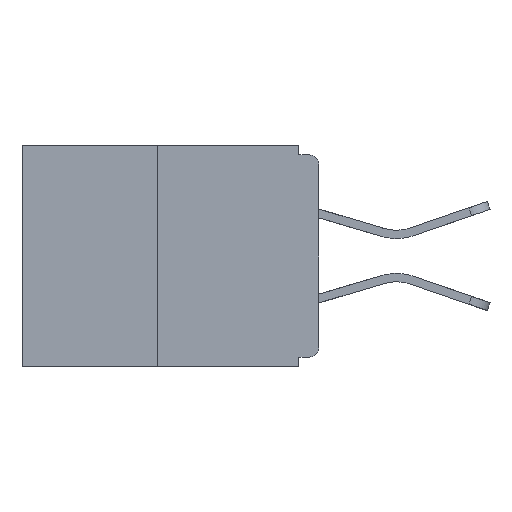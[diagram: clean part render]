
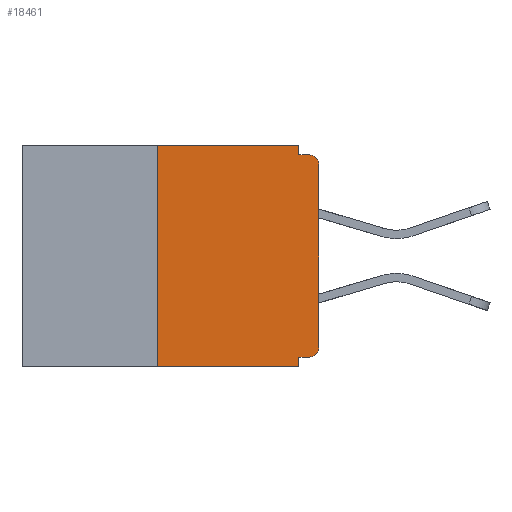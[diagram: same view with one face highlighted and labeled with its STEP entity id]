
A CAD part, left-side view. The second image highlights one B-rep face of the part: STEP entity #18461.
In plain terms, the highlighted planar face has unit normal (-1, 0, 0).
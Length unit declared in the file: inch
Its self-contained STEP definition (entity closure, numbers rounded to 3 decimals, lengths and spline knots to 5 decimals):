
#294 = VECTOR ( 'NONE', #12184, 39.37008 ) ;
#397 = VERTEX_POINT ( 'NONE', #10981 ) ;
#531 = CARTESIAN_POINT ( 'NONE',  ( 0., 0.46, -0.343 ) ) ;
#727 = LINE ( 'NONE', #11934, #294 ) ;
#805 = ORIENTED_EDGE ( 'NONE', *, *, #8348, .F. ) ;
#1010 = LINE ( 'NONE', #9107, #17300 ) ;
#1105 = DIRECTION ( 'NONE',  ( 0., 1., 0. ) ) ;
#1230 = DIRECTION ( 'NONE',  ( 0., 0., -1. ) ) ;
#1686 = DIRECTION ( 'NONE',  ( 0., 0., -1. ) ) ;
#1847 = ORIENTED_EDGE ( 'NONE', *, *, #14572, .F. ) ;
#2131 = ORIENTED_EDGE ( 'NONE', *, *, #13245, .F. ) ;
#2386 = VECTOR ( 'NONE', #1230, 39.37008 ) ;
#3093 = DIRECTION ( 'NONE',  ( 0., 0., -1. ) ) ;
#3113 = CARTESIAN_POINT ( 'NONE',  ( 0., 0.46, 0. ) ) ;
#3115 = VERTEX_POINT ( 'NONE', #5912 ) ;
#3250 = CARTESIAN_POINT ( 'NONE',  ( 0., 0.031, -0.015 ) ) ;
#3335 = VERTEX_POINT ( 'NONE', #14692 ) ;
#3386 = VERTEX_POINT ( 'NONE', #14561 ) ;
#3626 = VECTOR ( 'NONE', #14901, 39.37008 ) ;
#3733 = CARTESIAN_POINT ( 'NONE',  ( 0., 0.25, 0. ) ) ;
#4207 = LINE ( 'NONE', #9848, #2386 ) ;
#4228 = CIRCLE ( 'NONE', #4556, 0.015 ) ;
#4556 = AXIS2_PLACEMENT_3D ( 'NONE', #13564, #6342, #10470 ) ;
#4960 = DIRECTION ( 'NONE',  ( 0., -1., 0. ) ) ;
#5439 = VERTEX_POINT ( 'NONE', #5561 ) ;
#5561 = CARTESIAN_POINT ( 'NONE',  ( 0., 0.25, 0. ) ) ;
#5897 = EDGE_CURVE ( 'NONE', #17363, #3386, #16317, .T. ) ;
#5912 = CARTESIAN_POINT ( 'NONE',  ( 0., 0.015, -0.015 ) ) ;
#6247 = EDGE_CURVE ( 'NONE', #5439, #13983, #18509, .T. ) ;
#6342 = DIRECTION ( 'NONE',  ( -1., 0., 0. ) ) ;
#6622 = DIRECTION ( 'NONE',  ( 0., 0., 1. ) ) ;
#6623 = ORIENTED_EDGE ( 'NONE', *, *, #11339, .T. ) ;
#6711 = CARTESIAN_POINT ( 'NONE',  ( 0., 0.031, -0.328 ) ) ;
#6913 = VECTOR ( 'NONE', #1105, 39.37008 ) ;
#7054 = ORIENTED_EDGE ( 'NONE', *, *, #7511, .T. ) ;
#7511 = EDGE_CURVE ( 'NONE', #11652, #397, #8540, .T. ) ;
#8054 = CIRCLE ( 'NONE', #11321, 0.015 ) ;
#8132 = FACE_OUTER_BOUND ( 'NONE', #16042, .T. ) ;
#8278 = DIRECTION ( 'NONE',  ( 0., 0., 1. ) ) ;
#8348 = EDGE_CURVE ( 'NONE', #16678, #3115, #727, .T. ) ;
#8540 = LINE ( 'NONE', #531, #3626 ) ;
#8627 = CARTESIAN_POINT ( 'NONE',  ( 0., 0.015, -0.313 ) ) ;
#8867 = DIRECTION ( 'NONE',  ( -1., 0., 0. ) ) ;
#9107 = CARTESIAN_POINT ( 'NONE',  ( 0., 0.031, -0.343 ) ) ;
#9405 = EDGE_CURVE ( 'NONE', #11652, #5439, #13997, .T. ) ;
#9811 = CARTESIAN_POINT ( 'NONE',  ( 0., 0.25, -0.343 ) ) ;
#9848 = CARTESIAN_POINT ( 'NONE',  ( 0., 0.031, 0. ) ) ;
#10288 = PLANE ( 'NONE',  #15900 ) ;
#10373 = VECTOR ( 'NONE', #6622, 39.37008 ) ;
#10470 = DIRECTION ( 'NONE',  ( 0., 0., -1. ) ) ;
#10788 = ORIENTED_EDGE ( 'NONE', *, *, #14985, .F. ) ;
#10981 = CARTESIAN_POINT ( 'NONE',  ( 0., 0.031, -0.343 ) ) ;
#11066 = VECTOR ( 'NONE', #4960, 39.37008 ) ;
#11321 = AXIS2_PLACEMENT_3D ( 'NONE', #8627, #8867, #3093 ) ;
#11339 = EDGE_CURVE ( 'NONE', #3386, #3115, #4228, .T. ) ;
#11652 = VERTEX_POINT ( 'NONE', #9811 ) ;
#11829 = CARTESIAN_POINT ( 'NONE',  ( 0., 0., -0.313 ) ) ;
#11934 = CARTESIAN_POINT ( 'NONE',  ( 0., 0., -0.015 ) ) ;
#12066 = DIRECTION ( 'NONE',  ( 0., 0., -1. ) ) ;
#12184 = DIRECTION ( 'NONE',  ( 0., -1., 0. ) ) ;
#12320 = LINE ( 'NONE', #18198, #6913 ) ;
#13245 = EDGE_CURVE ( 'NONE', #13284, #397, #1010, .T. ) ;
#13284 = VERTEX_POINT ( 'NONE', #6711 ) ;
#13448 = ORIENTED_EDGE ( 'NONE', *, *, #13937, .T. ) ;
#13564 = CARTESIAN_POINT ( 'NONE',  ( 0., 0.015, -0.03 ) ) ;
#13580 = CARTESIAN_POINT ( 'NONE',  ( 0., 0.46, 0. ) ) ;
#13937 = EDGE_CURVE ( 'NONE', #3335, #17363, #8054, .T. ) ;
#13983 = VERTEX_POINT ( 'NONE', #15987 ) ;
#13997 = LINE ( 'NONE', #3733, #10373 ) ;
#14455 = DIRECTION ( 'NONE',  ( 1., 0., 0. ) ) ;
#14561 = CARTESIAN_POINT ( 'NONE',  ( 0., 0., -0.03 ) ) ;
#14572 = EDGE_CURVE ( 'NONE', #3335, #13284, #12320, .T. ) ;
#14692 = CARTESIAN_POINT ( 'NONE',  ( 0., 0.015, -0.328 ) ) ;
#14901 = DIRECTION ( 'NONE',  ( 0., -1., 0. ) ) ;
#14985 = EDGE_CURVE ( 'NONE', #13983, #16678, #4207, .T. ) ;
#15900 = AXIS2_PLACEMENT_3D ( 'NONE', #3113, #14455, #1686 ) ;
#15987 = CARTESIAN_POINT ( 'NONE',  ( 0., 0.031, 0. ) ) ;
#16042 = EDGE_LOOP ( 'NONE', ( #18150, #17155, #7054, #2131, #1847, #13448, #16691, #6623, #805, #10788 ) ) ;
#16317 = LINE ( 'NONE', #16919, #17429 ) ;
#16678 = VERTEX_POINT ( 'NONE', #3250 ) ;
#16691 = ORIENTED_EDGE ( 'NONE', *, *, #5897, .T. ) ;
#16919 = CARTESIAN_POINT ( 'NONE',  ( 0., 0., 0. ) ) ;
#17155 = ORIENTED_EDGE ( 'NONE', *, *, #9405, .F. ) ;
#17300 = VECTOR ( 'NONE', #12066, 39.37008 ) ;
#17363 = VERTEX_POINT ( 'NONE', #11829 ) ;
#17429 = VECTOR ( 'NONE', #8278, 39.37008 ) ;
#18150 = ORIENTED_EDGE ( 'NONE', *, *, #6247, .F. ) ;
#18198 = CARTESIAN_POINT ( 'NONE',  ( 0., 0., -0.328 ) ) ;
#18461 = ADVANCED_FACE ( 'NONE', ( #8132 ), #10288, .F. ) ;
#18509 = LINE ( 'NONE', #13580, #11066 ) ;
